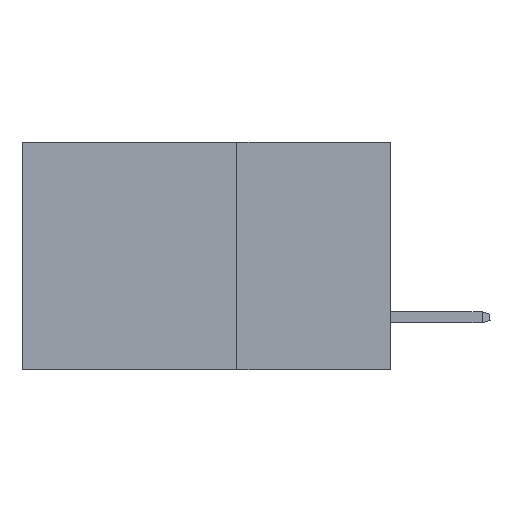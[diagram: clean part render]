
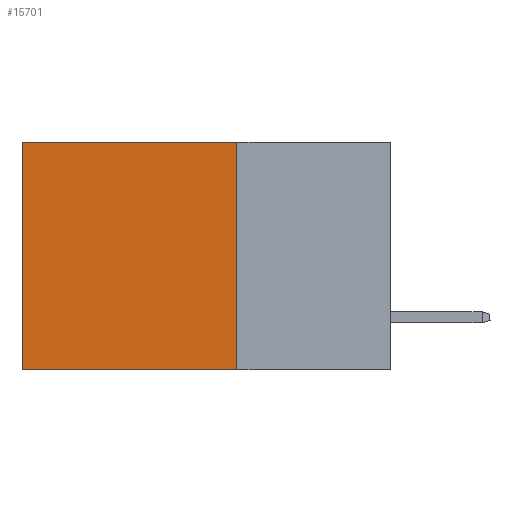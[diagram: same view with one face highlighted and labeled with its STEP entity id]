
A CAD part, left-side view. The second image highlights one B-rep face of the part: STEP entity #15701.
In plain terms, the highlighted planar face has unit normal (-1, 0, 0).
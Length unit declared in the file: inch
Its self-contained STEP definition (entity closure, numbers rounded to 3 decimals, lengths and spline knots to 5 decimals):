
#59 = VECTOR ( 'NONE', #1815, 39.37008 ) ;
#270 = AXIS2_PLACEMENT_3D ( 'NONE', #10555, #16344, #6540 ) ;
#330 = CARTESIAN_POINT ( 'NONE',  ( 0.2875, 0.25, -0.37 ) ) ;
#1815 = DIRECTION ( 'NONE',  ( 0., 1., 0. ) ) ;
#1960 = VERTEX_POINT ( 'NONE', #15500 ) ;
#2066 = CARTESIAN_POINT ( 'NONE',  ( 0.2875, 0.25, 0. ) ) ;
#3580 = LINE ( 'NONE', #330, #59 ) ;
#4908 = VECTOR ( 'NONE', #17448, 39.37008 ) ;
#5151 = ORIENTED_EDGE ( 'NONE', *, *, #7065, .T. ) ;
#5486 = CARTESIAN_POINT ( 'NONE',  ( 0.2875, 0.6, 0. ) ) ;
#5565 = CARTESIAN_POINT ( 'NONE',  ( 0.2875, 0.6, -0.37 ) ) ;
#6295 = FACE_OUTER_BOUND ( 'NONE', #10080, .T. ) ;
#6540 = DIRECTION ( 'NONE',  ( 0., 0., -1. ) ) ;
#6716 = EDGE_CURVE ( 'NONE', #1960, #15293, #3580, .T. ) ;
#7065 = EDGE_CURVE ( 'NONE', #16679, #17468, #14519, .T. ) ;
#7701 = VECTOR ( 'NONE', #9920, 39.37008 ) ;
#7902 = VECTOR ( 'NONE', #16749, 39.37008 ) ;
#9920 = DIRECTION ( 'NONE',  ( 0., 0., -1. ) ) ;
#10080 = EDGE_LOOP ( 'NONE', ( #16270, #11365, #14840, #5151 ) ) ;
#10555 = CARTESIAN_POINT ( 'NONE',  ( 0.2875, 0.25, 0. ) ) ;
#11270 = CARTESIAN_POINT ( 'NONE',  ( 0.2875, 0.25, 0. ) ) ;
#11365 = ORIENTED_EDGE ( 'NONE', *, *, #6716, .F. ) ;
#11450 = CARTESIAN_POINT ( 'NONE',  ( 0.2875, 0.25, 0. ) ) ;
#12000 = CARTESIAN_POINT ( 'NONE',  ( 0.2875, 0.6, 0. ) ) ;
#12044 = LINE ( 'NONE', #5486, #7902 ) ;
#12154 = PLANE ( 'NONE',  #270 ) ;
#12924 = LINE ( 'NONE', #11270, #7701 ) ;
#13561 = EDGE_CURVE ( 'NONE', #16679, #1960, #12924, .T. ) ;
#14013 = EDGE_CURVE ( 'NONE', #17468, #15293, #12044, .T. ) ;
#14519 = LINE ( 'NONE', #2066, #4908 ) ;
#14840 = ORIENTED_EDGE ( 'NONE', *, *, #13561, .F. ) ;
#15293 = VERTEX_POINT ( 'NONE', #5565 ) ;
#15500 = CARTESIAN_POINT ( 'NONE',  ( 0.2875, 0.25, -0.37 ) ) ;
#15701 = ADVANCED_FACE ( 'NONE', ( #6295 ), #12154, .F. ) ;
#16270 = ORIENTED_EDGE ( 'NONE', *, *, #14013, .T. ) ;
#16344 = DIRECTION ( 'NONE',  ( 1., 0., 0. ) ) ;
#16679 = VERTEX_POINT ( 'NONE', #11450 ) ;
#16749 = DIRECTION ( 'NONE',  ( 0., 0., -1. ) ) ;
#17448 = DIRECTION ( 'NONE',  ( 0., 1., 0. ) ) ;
#17468 = VERTEX_POINT ( 'NONE', #12000 ) ;
